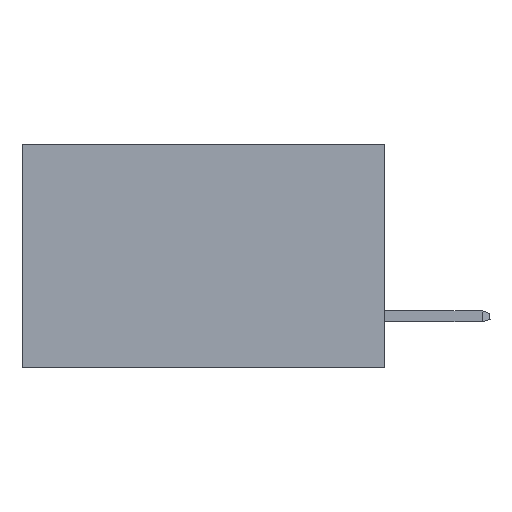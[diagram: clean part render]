
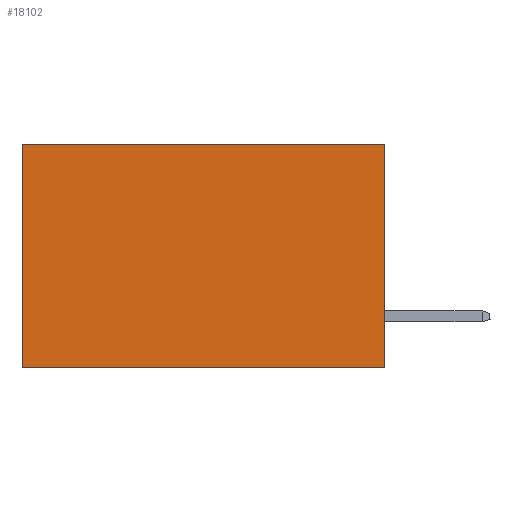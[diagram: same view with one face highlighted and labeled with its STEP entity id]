
A CAD part, left-side view. The second image highlights one B-rep face of the part: STEP entity #18102.
In plain terms, the highlighted planar face has unit normal (-1, 0, 0).
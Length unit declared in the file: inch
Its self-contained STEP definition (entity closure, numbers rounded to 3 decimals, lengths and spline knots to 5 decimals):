
#130 = EDGE_CURVE ( 'NONE', #15826, #16750, #2831, .T. ) ;
#401 = LINE ( 'NONE', #16710, #24505 ) ;
#540 = EDGE_CURVE ( 'NONE', #16750, #19150, #5090, .T. ) ;
#1208 = PLANE ( 'NONE',  #14012 ) ;
#1474 = DIRECTION ( 'NONE',  ( 1., 0., 0. ) ) ;
#1704 = ORIENTED_EDGE ( 'NONE', *, *, #1803, .F. ) ;
#1803 = EDGE_CURVE ( 'NONE', #15826, #23503, #401, .T. ) ;
#2162 = LINE ( 'NONE', #17968, #24345 ) ;
#2831 = LINE ( 'NONE', #12909, #7076 ) ;
#4783 = VECTOR ( 'NONE', #16631, 39.37008 ) ;
#5090 = LINE ( 'NONE', #16793, #4783 ) ;
#5396 = EDGE_LOOP ( 'NONE', ( #22047, #21089, #1704, #23360 ) ) ;
#5534 = CARTESIAN_POINT ( 'NONE',  ( 0.298, 0., 0. ) ) ;
#7076 = VECTOR ( 'NONE', #27312, 39.37008 ) ;
#11570 = CARTESIAN_POINT ( 'NONE',  ( 0.298, 0., 0. ) ) ;
#12909 = CARTESIAN_POINT ( 'NONE',  ( 0.298, 0., 0. ) ) ;
#14012 = AXIS2_PLACEMENT_3D ( 'NONE', #5534, #1474, #26659 ) ;
#15661 = CARTESIAN_POINT ( 'NONE',  ( 0.298, 0.6, -0.37 ) ) ;
#15826 = VERTEX_POINT ( 'NONE', #11570 ) ;
#16605 = DIRECTION ( 'NONE',  ( 0., 0., -1. ) ) ;
#16631 = DIRECTION ( 'NONE',  ( 0., 0., -1. ) ) ;
#16710 = CARTESIAN_POINT ( 'NONE',  ( 0.298, 0., 0. ) ) ;
#16750 = VERTEX_POINT ( 'NONE', #20066 ) ;
#16793 = CARTESIAN_POINT ( 'NONE',  ( 0.298, 0.6, 0. ) ) ;
#17968 = CARTESIAN_POINT ( 'NONE',  ( 0.298, 0., -0.37 ) ) ;
#18102 = ADVANCED_FACE ( 'NONE', ( #26135 ), #1208, .F. ) ;
#19150 = VERTEX_POINT ( 'NONE', #15661 ) ;
#20066 = CARTESIAN_POINT ( 'NONE',  ( 0.298, 0.6, 0. ) ) ;
#20687 = EDGE_CURVE ( 'NONE', #23503, #19150, #2162, .T. ) ;
#21089 = ORIENTED_EDGE ( 'NONE', *, *, #20687, .F. ) ;
#22047 = ORIENTED_EDGE ( 'NONE', *, *, #540, .T. ) ;
#22403 = DIRECTION ( 'NONE',  ( 0., 1., 0. ) ) ;
#23360 = ORIENTED_EDGE ( 'NONE', *, *, #130, .T. ) ;
#23503 = VERTEX_POINT ( 'NONE', #26009 ) ;
#24345 = VECTOR ( 'NONE', #22403, 39.37008 ) ;
#24505 = VECTOR ( 'NONE', #16605, 39.37008 ) ;
#26009 = CARTESIAN_POINT ( 'NONE',  ( 0.298, 0., -0.37 ) ) ;
#26135 = FACE_OUTER_BOUND ( 'NONE', #5396, .T. ) ;
#26659 = DIRECTION ( 'NONE',  ( 0., 0., -1. ) ) ;
#27312 = DIRECTION ( 'NONE',  ( 0., 1., 0. ) ) ;
